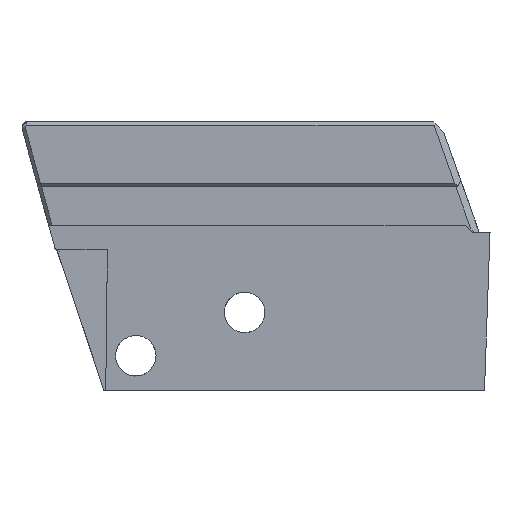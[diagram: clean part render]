
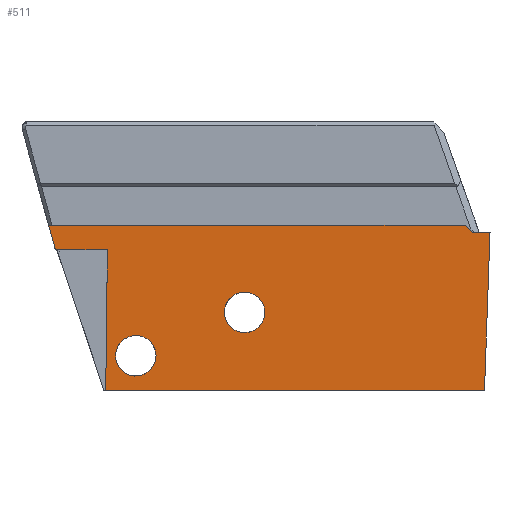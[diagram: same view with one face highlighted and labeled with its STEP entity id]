
A CAD part, front view. The second image highlights one B-rep face of the part: STEP entity #511.
In plain terms, the highlighted planar face has unit normal (0, -0.999, -0.035).
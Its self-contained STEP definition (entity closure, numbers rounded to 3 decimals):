
#48 = CARTESIAN_POINT ( 'NONE',  ( 0.542, 59.7, -6.559 ) ) ;
#63 = CARTESIAN_POINT ( 'NONE',  ( 0.542, 59.7, -6.559 ) ) ;
#142 = CARTESIAN_POINT ( 'NONE',  ( 0.542, 59.595, -3.559 ) ) ;
#169 = DIRECTION ( 'NONE',  ( 1., 0., 0. ) ) ;
#195 = CARTESIAN_POINT ( 'NONE',  ( -70.172, 59.474, -0.1 ) ) ;
#265 = CARTESIAN_POINT ( 'NONE',  ( -7.521, 59.707, -6.772 ) ) ;
#271 = LINE ( 'NONE', #1694, #477 ) ;
#298 =( BOUNDED_CURVE ( )  B_SPLINE_CURVE ( 3, ( #63, #4078, #2243, #2215 ),
 .UNSPECIFIED., .F., .T. ) 
 B_SPLINE_CURVE_WITH_KNOTS ( ( 4, 4 ),
 ( 4.712, 7.854 ),
 .UNSPECIFIED. ) 
 CURVE ( )  GEOMETRIC_REPRESENTATION_ITEM ( )  RATIONAL_B_SPLINE_CURVE ( ( 1., 0.333, 0.333, 1. ) ) 
 REPRESENTATION_ITEM ( '' )  );
#309 = EDGE_CURVE ( 'NONE', #3015, #1611, #2822, .T. ) ;
#313 = CARTESIAN_POINT ( 'NONE',  ( -7.521, 59.812, -9.772 ) ) ;
#399 = EDGE_CURVE ( 'NONE', #3571, #3015, #3452, .T. ) ;
#426 = CARTESIAN_POINT ( 'NONE',  ( -10.521, 59.917, -12.772 ) ) ;
#477 = VECTOR ( 'NONE', #3153, 1000. ) ;
#497 = ORIENTED_EDGE ( 'NONE', *, *, #745, .T. ) ;
#501 = FACE_BOUND ( 'NONE', #2336, .T. ) ;
#511 = ADVANCED_FACE ( 'NONE', ( #524, #501, #4466 ), #3115, .F. ) ;
#524 = FACE_BOUND ( 'NONE', #2268, .T. ) ;
#731 = ORIENTED_EDGE ( 'NONE', *, *, #399, .F. ) ;
#744 = ORIENTED_EDGE ( 'NONE', *, *, #1829, .F. ) ;
#745 = EDGE_CURVE ( 'NONE', #1672, #3650, #2262, .T. ) ;
#871 = CARTESIAN_POINT ( 'NONE',  ( -7.521, 59.812, -9.772 ) ) ;
#906 = DIRECTION ( 'NONE',  ( 0., 0.999, 0.035 ) ) ;
#952 = CARTESIAN_POINT ( 'NONE',  ( 17.207, 59.494, -0.654 ) ) ;
#1040 = VERTEX_POINT ( 'NONE', #2106 ) ;
#1175 = ORIENTED_EDGE ( 'NONE', *, *, #309, .F. ) ;
#1294 = LINE ( 'NONE', #4217, #3598 ) ;
#1326 = CARTESIAN_POINT ( 'NONE',  ( -10.521, 59.812, -9.772 ) ) ;
#1418 = VERTEX_POINT ( 'NONE', #4159 ) ;
#1435 = EDGE_CURVE ( 'NONE', #1040, #3831, #3391, .T. ) ;
#1445 = CARTESIAN_POINT ( 'NONE',  ( -7.521, 59.812, -9.772 ) ) ;
#1511 = DIRECTION ( 'NONE',  ( -1., 0., 0. ) ) ;
#1519 = CARTESIAN_POINT ( 'NONE',  ( 15.363, 59.474, -0.1 ) ) ;
#1611 = VERTEX_POINT ( 'NONE', #2527 ) ;
#1672 = VERTEX_POINT ( 'NONE', #871 ) ;
#1694 = CARTESIAN_POINT ( 'NONE',  ( -87.009, 59.494, -0.654 ) ) ;
#1829 = EDGE_CURVE ( 'NONE', #1611, #2860, #271, .T. ) ;
#1851 = CARTESIAN_POINT ( 'NONE',  ( 15.921, 59.494, -0.654 ) ) ;
#1856 = LINE ( 'NONE', #2569, #4531 ) ;
#1867 = CARTESIAN_POINT ( 'NONE',  ( -10.521, 59.812, -9.772 ) ) ;
#1877 = ORIENTED_EDGE ( 'NONE', *, *, #4179, .F. ) ;
#2003 = VECTOR ( 'NONE', #2320, 1000. ) ;
#2006 = DIRECTION ( 'NONE',  ( -0.266, -0.034, 0.963 ) ) ;
#2055 = CARTESIAN_POINT ( 'NONE',  ( -11.122, 59.539, -1.939 ) ) ;
#2065 = EDGE_CURVE ( 'NONE', #3650, #1672, #4556, .T. ) ;
#2106 = CARTESIAN_POINT ( 'NONE',  ( -2.458, 59.7, -6.559 ) ) ;
#2121 = ORIENTED_EDGE ( 'NONE', *, *, #4173, .T. ) ;
#2208 = DIRECTION ( 'NONE',  ( -1., 0., 0. ) ) ;
#2215 = CARTESIAN_POINT ( 'NONE',  ( -2.458, 59.7, -6.559 ) ) ;
#2243 = CARTESIAN_POINT ( 'NONE',  ( -2.458, 59.805, -9.559 ) ) ;
#2262 =( BOUNDED_CURVE ( )  B_SPLINE_CURVE ( 3, ( #1445, #3689, #426, #1867 ),
 .UNSPECIFIED., .F., .T. ) 
 B_SPLINE_CURVE_WITH_KNOTS ( ( 4, 4 ),
 ( 4.712, 7.854 ),
 .UNSPECIFIED. ) 
 CURVE ( )  GEOMETRIC_REPRESENTATION_ITEM ( )  RATIONAL_B_SPLINE_CURVE ( ( 1., 0.333, 0.333, 1. ) ) 
 REPRESENTATION_ITEM ( '' )  );
#2268 = EDGE_LOOP ( 'NONE', ( #3527, #497 ) ) ;
#2297 = CARTESIAN_POINT ( 'NONE',  ( 0.542, 59.7, -6.559 ) ) ;
#2320 = DIRECTION ( 'NONE',  ( 0.012, -0.035, 0.999 ) ) ;
#2327 = CARTESIAN_POINT ( 'NONE',  ( -15.472, 59.366, 2.998 ) ) ;
#2336 = EDGE_LOOP ( 'NONE', ( #2529, #2121 ) ) ;
#2464 = VERTEX_POINT ( 'NONE', #4080 ) ;
#2527 = CARTESIAN_POINT ( 'NONE',  ( 15.921, 59.494, -0.654 ) ) ;
#2529 = ORIENTED_EDGE ( 'NONE', *, *, #1435, .T. ) ;
#2569 = CARTESIAN_POINT ( 'NONE',  ( 32., 59.901, -12.321 ) ) ;
#2583 = ORIENTED_EDGE ( 'NONE', *, *, #3996, .F. ) ;
#2602 = EDGE_CURVE ( 'NONE', #2464, #2860, #1294, .T. ) ;
#2635 = CARTESIAN_POINT ( 'NONE',  ( 15.735, 59.487, -0.469 ) ) ;
#2688 = DIRECTION ( 'NONE',  ( 0.035, -0.035, 0.999 ) ) ;
#2717 = CARTESIAN_POINT ( 'NONE',  ( -2.458, 59.7, -6.559 ) ) ;
#2731 = CARTESIAN_POINT ( 'NONE',  ( -14.307, 59.622, -4.319 ) ) ;
#2748 = CARTESIAN_POINT ( 'NONE',  ( -10.521, 59.707, -6.772 ) ) ;
#2764 = CARTESIAN_POINT ( 'NONE',  ( -14.964, 59.539, -1.939 ) ) ;
#2779 = CARTESIAN_POINT ( 'NONE',  ( -15.472, 59.539, -1.939 ) ) ;
#2822 = B_SPLINE_CURVE_WITH_KNOTS ( 'NONE', 3,
 ( #4023, #4045, #2635, #1851 ),
 .UNSPECIFIED., .F., .F.,
 ( 4, 4 ),
 ( 0., 0.001 ),
 .UNSPECIFIED. ) ;
#2860 = VERTEX_POINT ( 'NONE', #952 ) ;
#3015 = VERTEX_POINT ( 'NONE', #1519 ) ;
#3097 = EDGE_CURVE ( 'NONE', #1418, #3139, #3347, .T. ) ;
#3115 = PLANE ( 'NONE',  #3448 ) ;
#3134 = CARTESIAN_POINT ( 'NONE',  ( -15.472, 59.474, -0.1 ) ) ;
#3139 = VERTEX_POINT ( 'NONE', #2055 ) ;
#3153 = DIRECTION ( 'NONE',  ( 1., 0., 0. ) ) ;
#3165 = EDGE_LOOP ( 'NONE', ( #1877, #3845, #744, #1175, #731, #2583, #3296, #4446 ) ) ;
#3172 = VECTOR ( 'NONE', #2208, 1000. ) ;
#3252 = VERTEX_POINT ( 'NONE', #2764 ) ;
#3296 = ORIENTED_EDGE ( 'NONE', *, *, #4477, .F. ) ;
#3347 = LINE ( 'NONE', #3707, #2003 ) ;
#3391 =( BOUNDED_CURVE ( )  B_SPLINE_CURVE ( 3, ( #2717, #4183, #142, #2297 ),
 .UNSPECIFIED., .F., .T. ) 
 B_SPLINE_CURVE_WITH_KNOTS ( ( 4, 4 ),
 ( 1.571, 4.712 ),
 .UNSPECIFIED. ) 
 CURVE ( )  GEOMETRIC_REPRESENTATION_ITEM ( )  RATIONAL_B_SPLINE_CURVE ( ( 1., 0.333, 0.333, 1. ) ) 
 REPRESENTATION_ITEM ( '' )  );
#3448 = AXIS2_PLACEMENT_3D ( 'NONE', #2327, #906, #4535 ) ;
#3452 = LINE ( 'NONE', #195, #3829 ) ;
#3527 = ORIENTED_EDGE ( 'NONE', *, *, #2065, .T. ) ;
#3571 = VERTEX_POINT ( 'NONE', #3134 ) ;
#3598 = VECTOR ( 'NONE', #2688, 1000. ) ;
#3643 = LINE ( 'NONE', #2779, #3172 ) ;
#3650 = VERTEX_POINT ( 'NONE', #1326 ) ;
#3689 = CARTESIAN_POINT ( 'NONE',  ( -7.521, 59.917, -12.772 ) ) ;
#3707 = CARTESIAN_POINT ( 'NONE',  ( -11.073, 59.394, 2.193 ) ) ;
#3829 = VECTOR ( 'NONE', #169, 1000. ) ;
#3831 = VERTEX_POINT ( 'NONE', #48 ) ;
#3845 = ORIENTED_EDGE ( 'NONE', *, *, #2602, .T. ) ;
#3910 = VECTOR ( 'NONE', #2006, 1000. ) ;
#3947 = CARTESIAN_POINT ( 'NONE',  ( -10.521, 59.812, -9.772 ) ) ;
#3996 = EDGE_CURVE ( 'NONE', #3252, #3571, #4220, .T. ) ;
#4023 = CARTESIAN_POINT ( 'NONE',  ( 15.363, 59.474, -0.1 ) ) ;
#4045 = CARTESIAN_POINT ( 'NONE',  ( 15.549, 59.481, -0.285 ) ) ;
#4078 = CARTESIAN_POINT ( 'NONE',  ( 0.542, 59.805, -9.559 ) ) ;
#4080 = CARTESIAN_POINT ( 'NONE',  ( 16.799, 59.901, -12.321 ) ) ;
#4159 = CARTESIAN_POINT ( 'NONE',  ( -11.243, 59.901, -12.321 ) ) ;
#4173 = EDGE_CURVE ( 'NONE', #3831, #1040, #298, .T. ) ;
#4179 = EDGE_CURVE ( 'NONE', #2464, #1418, #1856, .T. ) ;
#4183 = CARTESIAN_POINT ( 'NONE',  ( -2.458, 59.595, -3.559 ) ) ;
#4217 = CARTESIAN_POINT ( 'NONE',  ( 17.294, 59.406, 1.851 ) ) ;
#4220 = LINE ( 'NONE', #2731, #3910 ) ;
#4446 = ORIENTED_EDGE ( 'NONE', *, *, #3097, .F. ) ;
#4466 = FACE_OUTER_BOUND ( 'NONE', #3165, .T. ) ;
#4477 = EDGE_CURVE ( 'NONE', #3139, #3252, #3643, .T. ) ;
#4531 = VECTOR ( 'NONE', #1511, 1000. ) ;
#4535 = DIRECTION ( 'NONE',  ( 1., 0., 0. ) ) ;
#4556 =( BOUNDED_CURVE ( )  B_SPLINE_CURVE ( 3, ( #3947, #2748, #265, #313 ),
 .UNSPECIFIED., .F., .T. ) 
 B_SPLINE_CURVE_WITH_KNOTS ( ( 4, 4 ),
 ( 1.571, 4.712 ),
 .UNSPECIFIED. ) 
 CURVE ( )  GEOMETRIC_REPRESENTATION_ITEM ( )  RATIONAL_B_SPLINE_CURVE ( ( 1., 0.333, 0.333, 1. ) ) 
 REPRESENTATION_ITEM ( '' )  );
